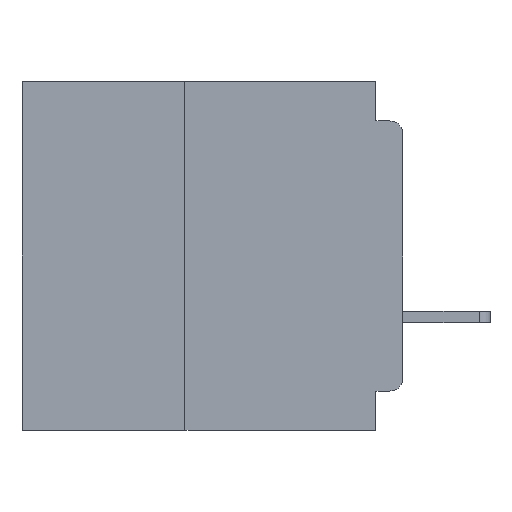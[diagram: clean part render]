
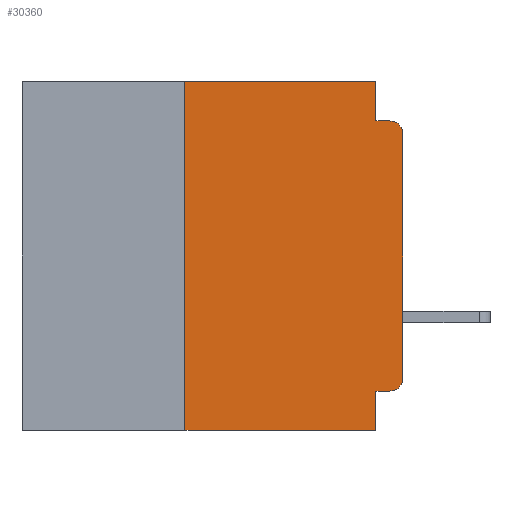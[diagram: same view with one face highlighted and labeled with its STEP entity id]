
A CAD part, left-side view. The second image highlights one B-rep face of the part: STEP entity #30360.
In plain terms, the highlighted planar face has unit normal (-1, 0, 0).
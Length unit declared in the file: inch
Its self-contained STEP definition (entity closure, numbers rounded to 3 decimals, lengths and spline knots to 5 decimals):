
#143 = AXIS2_PLACEMENT_3D ( 'NONE', #12275, #16934, #49345 ) ;
#1947 = DIRECTION ( 'NONE',  ( 0., 0., 1. ) ) ;
#2111 = LINE ( 'NONE', #8242, #15977 ) ;
#2685 = PLANE ( 'NONE',  #143 ) ;
#6441 = CARTESIAN_POINT ( 'NONE',  ( 0., 0., 0. ) ) ;
#6907 = EDGE_CURVE ( 'NONE', #49366, #27627, #56563, .T. ) ;
#6952 = VECTOR ( 'NONE', #12692, 39.37008 ) ;
#8005 = CARTESIAN_POINT ( 'NONE',  ( 0., 0.437, 0. ) ) ;
#8242 = CARTESIAN_POINT ( 'NONE',  ( 0., 0., -0.045 ) ) ;
#8507 = LINE ( 'NONE', #27442, #56301 ) ;
#8744 = ORIENTED_EDGE ( 'NONE', *, *, #29792, .F. ) ;
#9363 = ORIENTED_EDGE ( 'NONE', *, *, #13251, .F. ) ;
#9653 = EDGE_CURVE ( 'NONE', #58185, #16369, #59778, .T. ) ;
#12275 = CARTESIAN_POINT ( 'NONE',  ( 0., 0.437, 0. ) ) ;
#12506 = DIRECTION ( 'NONE',  ( 0., 0., 1. ) ) ;
#12692 = DIRECTION ( 'NONE',  ( 0., -1., 0. ) ) ;
#12867 = LINE ( 'NONE', #54028, #59148 ) ;
#13251 = EDGE_CURVE ( 'NONE', #24661, #56134, #34859, .T. ) ;
#15977 = VECTOR ( 'NONE', #40695, 39.37008 ) ;
#16317 = CARTESIAN_POINT ( 'NONE',  ( 0., 0.015, -0.34 ) ) ;
#16369 = VERTEX_POINT ( 'NONE', #40890 ) ;
#16731 = DIRECTION ( 'NONE',  ( 0., 1., 0. ) ) ;
#16934 = DIRECTION ( 'NONE',  ( 1., 0., 0. ) ) ;
#18182 = DIRECTION ( 'NONE',  ( 0., 0., -1. ) ) ;
#19173 = VECTOR ( 'NONE', #40112, 39.37008 ) ;
#19307 = DIRECTION ( 'NONE',  ( -1., 0., 0. ) ) ;
#21000 = DIRECTION ( 'NONE',  ( 0., 0., -1. ) ) ;
#21305 = FACE_OUTER_BOUND ( 'NONE', #50738, .T. ) ;
#21442 = LINE ( 'NONE', #53770, #58280 ) ;
#21728 = CARTESIAN_POINT ( 'NONE',  ( 0., 0.25, -0.4 ) ) ;
#22570 = ORIENTED_EDGE ( 'NONE', *, *, #40950, .F. ) ;
#23099 = EDGE_CURVE ( 'NONE', #51011, #56134, #8507, .T. ) ;
#23812 = ORIENTED_EDGE ( 'NONE', *, *, #6907, .T. ) ;
#24447 = CARTESIAN_POINT ( 'NONE',  ( 0., 0.015, -0.045 ) ) ;
#24661 = VERTEX_POINT ( 'NONE', #46697 ) ;
#26179 = LINE ( 'NONE', #6441, #38473 ) ;
#26801 = CARTESIAN_POINT ( 'NONE',  ( 0., 0.031, 0. ) ) ;
#27442 = CARTESIAN_POINT ( 'NONE',  ( 0., 0.437, -0.4 ) ) ;
#27627 = VERTEX_POINT ( 'NONE', #24447 ) ;
#28379 = CARTESIAN_POINT ( 'NONE',  ( 0., 0., -0.06 ) ) ;
#28754 = ORIENTED_EDGE ( 'NONE', *, *, #49717, .F. ) ;
#29792 = EDGE_CURVE ( 'NONE', #41659, #49790, #56074, .T. ) ;
#30360 = ADVANCED_FACE ( 'NONE', ( #21305 ), #2685, .F. ) ;
#31653 = LINE ( 'NONE', #8005, #6952 ) ;
#32501 = ORIENTED_EDGE ( 'NONE', *, *, #23099, .T. ) ;
#32528 = ORIENTED_EDGE ( 'NONE', *, *, #40354, .F. ) ;
#34697 = AXIS2_PLACEMENT_3D ( 'NONE', #47050, #19307, #51720 ) ;
#34859 = LINE ( 'NONE', #41292, #57944 ) ;
#34924 = ORIENTED_EDGE ( 'NONE', *, *, #9653, .T. ) ;
#37339 = CARTESIAN_POINT ( 'NONE',  ( 0., 0.25, 0. ) ) ;
#38473 = VECTOR ( 'NONE', #1947, 39.37008 ) ;
#40112 = DIRECTION ( 'NONE',  ( 0., 0., -1. ) ) ;
#40354 = EDGE_CURVE ( 'NONE', #47955, #41659, #31653, .T. ) ;
#40695 = DIRECTION ( 'NONE',  ( 0., -1., 0. ) ) ;
#40890 = CARTESIAN_POINT ( 'NONE',  ( 0., 0., -0.34 ) ) ;
#40950 = EDGE_CURVE ( 'NONE', #58185, #24661, #21442, .T. ) ;
#41292 = CARTESIAN_POINT ( 'NONE',  ( 0., 0.031, -0.4 ) ) ;
#41395 = DIRECTION ( 'NONE',  ( 0., -1., 0. ) ) ;
#41659 = VERTEX_POINT ( 'NONE', #26801 ) ;
#42841 = ORIENTED_EDGE ( 'NONE', *, *, #48182, .T. ) ;
#44942 = CARTESIAN_POINT ( 'NONE',  ( 0., 0.031, 0. ) ) ;
#45307 = CARTESIAN_POINT ( 'NONE',  ( 0., 0.031, -0.045 ) ) ;
#46697 = CARTESIAN_POINT ( 'NONE',  ( 0., 0.031, -0.355 ) ) ;
#47050 = CARTESIAN_POINT ( 'NONE',  ( 0., 0.015, -0.06 ) ) ;
#47955 = VERTEX_POINT ( 'NONE', #37339 ) ;
#48182 = EDGE_CURVE ( 'NONE', #16369, #49366, #26179, .T. ) ;
#48418 = EDGE_CURVE ( 'NONE', #49790, #27627, #2111, .T. ) ;
#48724 = DIRECTION ( 'NONE',  ( -1., 0., 0. ) ) ;
#48758 = CARTESIAN_POINT ( 'NONE',  ( 0., 0.031, -0.4 ) ) ;
#49087 = CARTESIAN_POINT ( 'NONE',  ( 0., 0.015, -0.355 ) ) ;
#49153 = AXIS2_PLACEMENT_3D ( 'NONE', #16317, #48724, #21000 ) ;
#49345 = DIRECTION ( 'NONE',  ( 0., 0., -1. ) ) ;
#49366 = VERTEX_POINT ( 'NONE', #28379 ) ;
#49717 = EDGE_CURVE ( 'NONE', #51011, #47955, #12867, .T. ) ;
#49790 = VERTEX_POINT ( 'NONE', #45307 ) ;
#50738 = EDGE_LOOP ( 'NONE', ( #42841, #23812, #58493, #8744, #32528, #28754, #32501, #9363, #22570, #34924 ) ) ;
#51011 = VERTEX_POINT ( 'NONE', #21728 ) ;
#51720 = DIRECTION ( 'NONE',  ( 0., 0., -1. ) ) ;
#53770 = CARTESIAN_POINT ( 'NONE',  ( 0., 0., -0.355 ) ) ;
#54028 = CARTESIAN_POINT ( 'NONE',  ( 0., 0.25, -0.4 ) ) ;
#56074 = LINE ( 'NONE', #44942, #19173 ) ;
#56134 = VERTEX_POINT ( 'NONE', #48758 ) ;
#56301 = VECTOR ( 'NONE', #41395, 39.37008 ) ;
#56563 = CIRCLE ( 'NONE', #34697, 0.015 ) ;
#57944 = VECTOR ( 'NONE', #18182, 39.37008 ) ;
#58185 = VERTEX_POINT ( 'NONE', #49087 ) ;
#58280 = VECTOR ( 'NONE', #16731, 39.37008 ) ;
#58493 = ORIENTED_EDGE ( 'NONE', *, *, #48418, .F. ) ;
#59148 = VECTOR ( 'NONE', #12506, 39.37008 ) ;
#59778 = CIRCLE ( 'NONE', #49153, 0.015 ) ;
